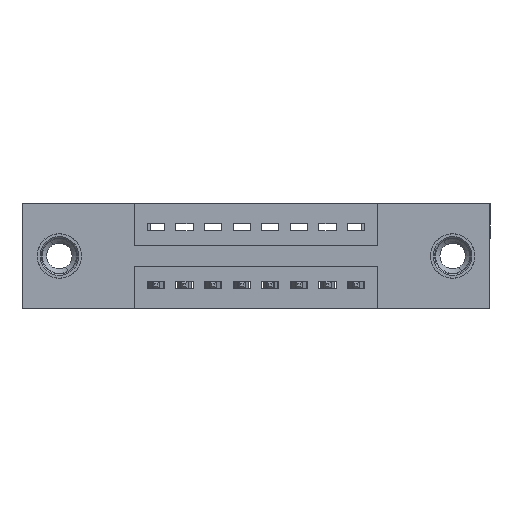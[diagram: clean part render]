
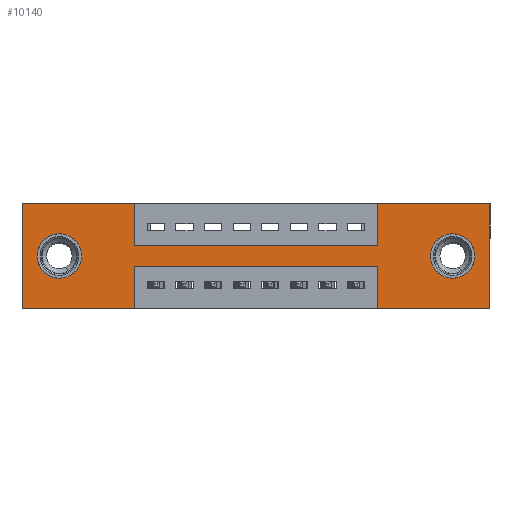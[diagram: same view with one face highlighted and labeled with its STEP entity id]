
A CAD part, front view. The second image highlights one B-rep face of the part: STEP entity #10140.
In plain terms, the highlighted planar face has unit normal (0, -1, 0).
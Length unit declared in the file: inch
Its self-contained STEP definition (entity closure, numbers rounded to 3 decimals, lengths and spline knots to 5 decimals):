
#61 = CARTESIAN_POINT ( 'NONE',  ( 0.13, 0., -0.263 ) ) ;
#179 = EDGE_CURVE ( 'NONE', #12313, #12153, #11841, .T. ) ;
#244 = CARTESIAN_POINT ( 'NONE',  ( 0., 0., -0.37 ) ) ;
#322 = DIRECTION ( 'NONE',  ( 0., 0., 1. ) ) ;
#455 = CARTESIAN_POINT ( 'NONE',  ( 0., 0., -0.37 ) ) ;
#551 = FACE_OUTER_BOUND ( 'NONE', #813, .T. ) ;
#596 = EDGE_CURVE ( 'NONE', #5246, #4055, #1602, .T. ) ;
#674 = LINE ( 'NONE', #244, #3828 ) ;
#813 = EDGE_LOOP ( 'NONE', ( #10302, #8607, #9419, #6777, #4014, #8533, #4254, #12384, #13812, #3765, #10183, #14908 ) ) ;
#1224 = CARTESIAN_POINT ( 'NONE',  ( 1.635, 0., -0.37 ) ) ;
#1602 = LINE ( 'NONE', #14053, #11078 ) ;
#1721 = DIRECTION ( 'NONE',  ( 1., 0., 0. ) ) ;
#1850 = ORIENTED_EDGE ( 'NONE', *, *, #14761, .T. ) ;
#1988 = VECTOR ( 'NONE', #1721, 39.37008 ) ;
#2089 = VECTOR ( 'NONE', #5569, 39.37008 ) ;
#2584 = AXIS2_PLACEMENT_3D ( 'NONE', #3934, #6373, #322 ) ;
#2723 = DIRECTION ( 'NONE',  ( 0., -1., 0. ) ) ;
#2823 = CARTESIAN_POINT ( 'NONE',  ( 1.635, 0., 0. ) ) ;
#2910 = CARTESIAN_POINT ( 'NONE',  ( 0.3925, 0., -0.22 ) ) ;
#2949 = DIRECTION ( 'NONE',  ( 0., 1., 0. ) ) ;
#3280 = AXIS2_PLACEMENT_3D ( 'NONE', #9400, #4568, #10476 ) ;
#3765 = ORIENTED_EDGE ( 'NONE', *, *, #7642, .F. ) ;
#3828 = VECTOR ( 'NONE', #8535, 39.37008 ) ;
#3934 = CARTESIAN_POINT ( 'NONE',  ( 0.13, 0., -0.185 ) ) ;
#3977 = CARTESIAN_POINT ( 'NONE',  ( 0., 0., 0. ) ) ;
#4014 = ORIENTED_EDGE ( 'NONE', *, *, #6469, .F. ) ;
#4023 = DIRECTION ( 'NONE',  ( 0., 0., -1. ) ) ;
#4055 = VERTEX_POINT ( 'NONE', #15247 ) ;
#4079 = CARTESIAN_POINT ( 'NONE',  ( 0., 0., 0. ) ) ;
#4133 = CIRCLE ( 'NONE', #13311, 0.078 ) ;
#4254 = ORIENTED_EDGE ( 'NONE', *, *, #596, .F. ) ;
#4449 = CARTESIAN_POINT ( 'NONE',  ( 0.3925, 0., 0. ) ) ;
#4568 = DIRECTION ( 'NONE',  ( 0., 1., 0. ) ) ;
#4826 = CARTESIAN_POINT ( 'NONE',  ( 1.2425, 0., -0.22 ) ) ;
#5142 = EDGE_CURVE ( 'NONE', #7324, #13723, #7590, .T. ) ;
#5246 = VERTEX_POINT ( 'NONE', #12115 ) ;
#5296 = DIRECTION ( 'NONE',  ( 0., 0., 1. ) ) ;
#5319 = CARTESIAN_POINT ( 'NONE',  ( 0.3925, 0., 0. ) ) ;
#5541 = VECTOR ( 'NONE', #8323, 39.37008 ) ;
#5551 = EDGE_CURVE ( 'NONE', #12915, #5246, #8144, .T. ) ;
#5569 = DIRECTION ( 'NONE',  ( 0., 0., 1. ) ) ;
#5726 = DIRECTION ( 'NONE',  ( 0., 0., 1. ) ) ;
#5929 = FACE_BOUND ( 'NONE', #7229, .T. ) ;
#6237 = CARTESIAN_POINT ( 'NONE',  ( 0., 0., 0. ) ) ;
#6276 = PLANE ( 'NONE',  #12229 ) ;
#6302 = VERTEX_POINT ( 'NONE', #455 ) ;
#6373 = DIRECTION ( 'NONE',  ( 0., 1., 0. ) ) ;
#6469 = EDGE_CURVE ( 'NONE', #12807, #6936, #8662, .T. ) ;
#6637 = EDGE_CURVE ( 'NONE', #4055, #12807, #9941, .T. ) ;
#6650 = CARTESIAN_POINT ( 'NONE',  ( 0.13, 0., -0.185 ) ) ;
#6777 = ORIENTED_EDGE ( 'NONE', *, *, #6807, .F. ) ;
#6795 = VECTOR ( 'NONE', #7577, 39.37008 ) ;
#6807 = EDGE_CURVE ( 'NONE', #6936, #13431, #674, .T. ) ;
#6821 = CARTESIAN_POINT ( 'NONE',  ( 0.3925, 0., -0.37 ) ) ;
#6936 = VERTEX_POINT ( 'NONE', #1224 ) ;
#6950 = VECTOR ( 'NONE', #12698, 39.37008 ) ;
#7229 = EDGE_LOOP ( 'NONE', ( #11780, #13393 ) ) ;
#7324 = VERTEX_POINT ( 'NONE', #4826 ) ;
#7484 = CARTESIAN_POINT ( 'NONE',  ( 0., 0., -0.37 ) ) ;
#7558 = DIRECTION ( 'NONE',  ( 0., 0., -1. ) ) ;
#7577 = DIRECTION ( 'NONE',  ( 1., 0., 0. ) ) ;
#7590 = LINE ( 'NONE', #14200, #5541 ) ;
#7642 = EDGE_CURVE ( 'NONE', #10696, #10790, #10084, .T. ) ;
#7870 = VECTOR ( 'NONE', #13495, 39.37008 ) ;
#7899 = VECTOR ( 'NONE', #7558, 39.37008 ) ;
#7912 = CARTESIAN_POINT ( 'NONE',  ( 1.2425, 0., -0.37 ) ) ;
#7937 = EDGE_CURVE ( 'NONE', #13431, #7324, #11554, .T. ) ;
#7962 = VECTOR ( 'NONE', #13990, 39.37008 ) ;
#8144 = LINE ( 'NONE', #8850, #1988 ) ;
#8323 = DIRECTION ( 'NONE',  ( -1., 0., 0. ) ) ;
#8473 = VECTOR ( 'NONE', #4023, 39.37008 ) ;
#8533 = ORIENTED_EDGE ( 'NONE', *, *, #6637, .F. ) ;
#8535 = DIRECTION ( 'NONE',  ( -1., 0., 0. ) ) ;
#8607 = ORIENTED_EDGE ( 'NONE', *, *, #5142, .F. ) ;
#8627 = CARTESIAN_POINT ( 'NONE',  ( 1.505, 0., -0.263 ) ) ;
#8644 = LINE ( 'NONE', #5319, #7899 ) ;
#8662 = LINE ( 'NONE', #2823, #8473 ) ;
#8850 = CARTESIAN_POINT ( 'NONE',  ( 0.3925, 0., -0.15 ) ) ;
#8875 = VERTEX_POINT ( 'NONE', #9891 ) ;
#9069 = VECTOR ( 'NONE', #5296, 39.37008 ) ;
#9098 = VERTEX_POINT ( 'NONE', #11343 ) ;
#9400 = CARTESIAN_POINT ( 'NONE',  ( 1.505, 0., -0.185 ) ) ;
#9419 = ORIENTED_EDGE ( 'NONE', *, *, #7937, .F. ) ;
#9429 = CARTESIAN_POINT ( 'NONE',  ( 1.2425, 0., -0.37 ) ) ;
#9560 = DIRECTION ( 'NONE',  ( 0., 0., -1. ) ) ;
#9733 = EDGE_CURVE ( 'NONE', #12805, #9098, #13027, .T. ) ;
#9891 = CARTESIAN_POINT ( 'NONE',  ( 0.3925, 0., -0.37 ) ) ;
#9941 = LINE ( 'NONE', #3977, #6795 ) ;
#10084 = LINE ( 'NONE', #15025, #6950 ) ;
#10140 = ADVANCED_FACE ( 'NONE', ( #11311, #5929, #551 ), #6276, .T. ) ;
#10183 = ORIENTED_EDGE ( 'NONE', *, *, #11113, .F. ) ;
#10302 = ORIENTED_EDGE ( 'NONE', *, *, #12031, .F. ) ;
#10476 = DIRECTION ( 'NONE',  ( 0., 0., -1. ) ) ;
#10696 = VERTEX_POINT ( 'NONE', #6237 ) ;
#10790 = VERTEX_POINT ( 'NONE', #4449 ) ;
#10911 = LINE ( 'NONE', #6821, #7962 ) ;
#11078 = VECTOR ( 'NONE', #5726, 39.37008 ) ;
#11113 = EDGE_CURVE ( 'NONE', #6302, #10696, #12233, .T. ) ;
#11201 = DIRECTION ( 'NONE',  ( 0., 1., 0. ) ) ;
#11222 = EDGE_LOOP ( 'NONE', ( #1850, #13302 ) ) ;
#11311 = FACE_BOUND ( 'NONE', #11222, .T. ) ;
#11343 = CARTESIAN_POINT ( 'NONE',  ( 0.13, 0., -0.107 ) ) ;
#11459 = DIRECTION ( 'NONE',  ( 0., 0., 1. ) ) ;
#11554 = LINE ( 'NONE', #7912, #2089 ) ;
#11780 = ORIENTED_EDGE ( 'NONE', *, *, #12905, .T. ) ;
#11841 = CIRCLE ( 'NONE', #3280, 0.078 ) ;
#12031 = EDGE_CURVE ( 'NONE', #13723, #8875, #10911, .T. ) ;
#12041 = CARTESIAN_POINT ( 'NONE',  ( 1.635, 0., 0. ) ) ;
#12115 = CARTESIAN_POINT ( 'NONE',  ( 1.2425, 0., -0.15 ) ) ;
#12153 = VERTEX_POINT ( 'NONE', #14296 ) ;
#12229 = AXIS2_PLACEMENT_3D ( 'NONE', #7484, #2723, #13218 ) ;
#12233 = LINE ( 'NONE', #4079, #9069 ) ;
#12313 = VERTEX_POINT ( 'NONE', #8627 ) ;
#12333 = CARTESIAN_POINT ( 'NONE',  ( 0.3925, 0., -0.15 ) ) ;
#12365 = CIRCLE ( 'NONE', #2584, 0.078 ) ;
#12384 = ORIENTED_EDGE ( 'NONE', *, *, #5551, .F. ) ;
#12571 = CARTESIAN_POINT ( 'NONE',  ( 1.505, 0., -0.185 ) ) ;
#12698 = DIRECTION ( 'NONE',  ( 1., 0., 0. ) ) ;
#12805 = VERTEX_POINT ( 'NONE', #61 ) ;
#12807 = VERTEX_POINT ( 'NONE', #12041 ) ;
#12905 = EDGE_CURVE ( 'NONE', #9098, #12805, #12365, .T. ) ;
#12915 = VERTEX_POINT ( 'NONE', #12333 ) ;
#13027 = CIRCLE ( 'NONE', #14898, 0.078 ) ;
#13218 = DIRECTION ( 'NONE',  ( 0., 0., -1. ) ) ;
#13302 = ORIENTED_EDGE ( 'NONE', *, *, #179, .T. ) ;
#13311 = AXIS2_PLACEMENT_3D ( 'NONE', #12571, #11201, #9560 ) ;
#13393 = ORIENTED_EDGE ( 'NONE', *, *, #9733, .T. ) ;
#13431 = VERTEX_POINT ( 'NONE', #9429 ) ;
#13495 = DIRECTION ( 'NONE',  ( -1., 0., 0. ) ) ;
#13709 = EDGE_CURVE ( 'NONE', #10790, #12915, #8644, .T. ) ;
#13723 = VERTEX_POINT ( 'NONE', #2910 ) ;
#13812 = ORIENTED_EDGE ( 'NONE', *, *, #13709, .F. ) ;
#13990 = DIRECTION ( 'NONE',  ( 0., 0., -1. ) ) ;
#14001 = LINE ( 'NONE', #14754, #7870 ) ;
#14053 = CARTESIAN_POINT ( 'NONE',  ( 1.2425, 0., 0. ) ) ;
#14200 = CARTESIAN_POINT ( 'NONE',  ( 0.3925, 0., -0.22 ) ) ;
#14296 = CARTESIAN_POINT ( 'NONE',  ( 1.505, 0., -0.107 ) ) ;
#14742 = EDGE_CURVE ( 'NONE', #8875, #6302, #14001, .T. ) ;
#14754 = CARTESIAN_POINT ( 'NONE',  ( 0., 0., -0.37 ) ) ;
#14761 = EDGE_CURVE ( 'NONE', #12153, #12313, #4133, .T. ) ;
#14898 = AXIS2_PLACEMENT_3D ( 'NONE', #6650, #2949, #11459 ) ;
#14908 = ORIENTED_EDGE ( 'NONE', *, *, #14742, .F. ) ;
#15025 = CARTESIAN_POINT ( 'NONE',  ( 0., 0., 0. ) ) ;
#15247 = CARTESIAN_POINT ( 'NONE',  ( 1.2425, 0., 0. ) ) ;
